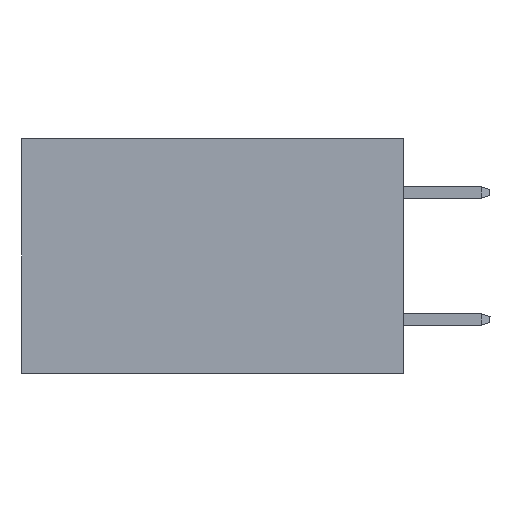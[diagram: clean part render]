
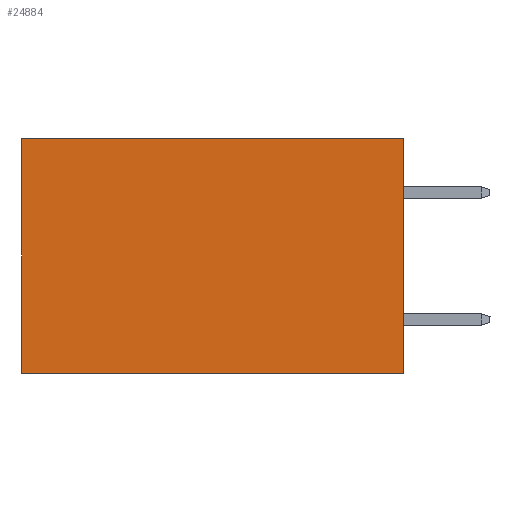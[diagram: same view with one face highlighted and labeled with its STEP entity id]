
A CAD part, left-side view. The second image highlights one B-rep face of the part: STEP entity #24884.
In plain terms, the highlighted planar face has unit normal (-1, 0, 0).
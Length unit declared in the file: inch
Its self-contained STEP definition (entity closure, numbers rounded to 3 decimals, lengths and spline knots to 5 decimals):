
#29 = VERTEX_POINT ( 'NONE', #26055 ) ;
#101 = VERTEX_POINT ( 'NONE', #17531 ) ;
#350 = LINE ( 'NONE', #10274, #5337 ) ;
#1055 = ORIENTED_EDGE ( 'NONE', *, *, #8980, .F. ) ;
#4761 = VECTOR ( 'NONE', #26919, 39.37008 ) ;
#5337 = VECTOR ( 'NONE', #7827, 39.37008 ) ;
#6257 = DIRECTION ( 'NONE',  ( 0., 0., -1. ) ) ;
#7827 = DIRECTION ( 'NONE',  ( 0., 0., -1. ) ) ;
#8664 = VECTOR ( 'NONE', #27444, 39.37008 ) ;
#8980 = EDGE_CURVE ( 'NONE', #21630, #101, #350, .T. ) ;
#10274 = CARTESIAN_POINT ( 'NONE',  ( 0.2875, 0., 0. ) ) ;
#10954 = CARTESIAN_POINT ( 'NONE',  ( 0.2875, 0., 0. ) ) ;
#11337 = CARTESIAN_POINT ( 'NONE',  ( 0.2875, 0., 0. ) ) ;
#12690 = EDGE_CURVE ( 'NONE', #21630, #29, #16078, .T. ) ;
#14354 = EDGE_CURVE ( 'NONE', #101, #28154, #14567, .T. ) ;
#14567 = LINE ( 'NONE', #14896, #8664 ) ;
#14896 = CARTESIAN_POINT ( 'NONE',  ( 0.2875, 0., -0.37 ) ) ;
#16078 = LINE ( 'NONE', #11337, #4761 ) ;
#16487 = EDGE_LOOP ( 'NONE', ( #25784, #24824, #1055, #30400 ) ) ;
#17531 = CARTESIAN_POINT ( 'NONE',  ( 0.2875, 0., -0.37 ) ) ;
#17908 = EDGE_CURVE ( 'NONE', #29, #28154, #25823, .T. ) ;
#17965 = FACE_OUTER_BOUND ( 'NONE', #16487, .T. ) ;
#18625 = DIRECTION ( 'NONE',  ( 1., 0., 0. ) ) ;
#21089 = CARTESIAN_POINT ( 'NONE',  ( 0.2875, 0.6, 0. ) ) ;
#21300 = CARTESIAN_POINT ( 'NONE',  ( 0.2875, 0., 0. ) ) ;
#21630 = VERTEX_POINT ( 'NONE', #21300 ) ;
#21948 = VECTOR ( 'NONE', #6257, 39.37008 ) ;
#24824 = ORIENTED_EDGE ( 'NONE', *, *, #14354, .F. ) ;
#24884 = ADVANCED_FACE ( 'NONE', ( #17965 ), #25781, .F. ) ;
#25781 = PLANE ( 'NONE',  #28034 ) ;
#25784 = ORIENTED_EDGE ( 'NONE', *, *, #17908, .T. ) ;
#25823 = LINE ( 'NONE', #21089, #21948 ) ;
#26055 = CARTESIAN_POINT ( 'NONE',  ( 0.2875, 0.6, 0. ) ) ;
#26642 = CARTESIAN_POINT ( 'NONE',  ( 0.2875, 0.6, -0.37 ) ) ;
#26919 = DIRECTION ( 'NONE',  ( 0., 1., 0. ) ) ;
#27444 = DIRECTION ( 'NONE',  ( 0., 1., 0. ) ) ;
#27902 = DIRECTION ( 'NONE',  ( 0., 0., -1. ) ) ;
#28034 = AXIS2_PLACEMENT_3D ( 'NONE', #10954, #18625, #27902 ) ;
#28154 = VERTEX_POINT ( 'NONE', #26642 ) ;
#30400 = ORIENTED_EDGE ( 'NONE', *, *, #12690, .T. ) ;
